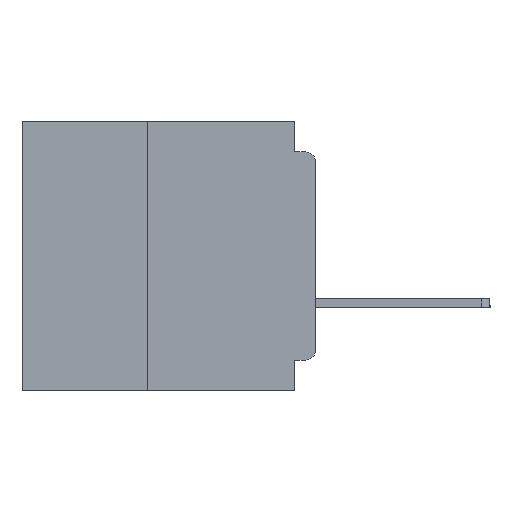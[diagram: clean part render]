
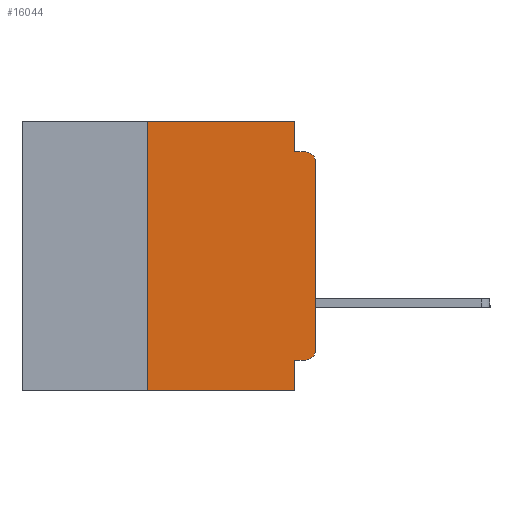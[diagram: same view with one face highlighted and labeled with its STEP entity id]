
A CAD part, left-side view. The second image highlights one B-rep face of the part: STEP entity #16044.
In plain terms, the highlighted planar face has unit normal (-1, 0, 0).
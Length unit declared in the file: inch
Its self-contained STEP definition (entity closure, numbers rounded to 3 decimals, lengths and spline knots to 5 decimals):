
#1748 = VECTOR ( 'NONE', #27761, 39.37008 ) ;
#2003 = CARTESIAN_POINT ( 'NONE',  ( 0., 0., -0.06 ) ) ;
#2313 = CARTESIAN_POINT ( 'NONE',  ( 0., 0.031, -0.4 ) ) ;
#3567 = VERTEX_POINT ( 'NONE', #19985 ) ;
#4343 = VECTOR ( 'NONE', #8860, 39.37008 ) ;
#4599 = VECTOR ( 'NONE', #20821, 39.37008 ) ;
#5480 = VERTEX_POINT ( 'NONE', #22633 ) ;
#5683 = LINE ( 'NONE', #7481, #4599 ) ;
#5689 = VERTEX_POINT ( 'NONE', #27144 ) ;
#6743 = DIRECTION ( 'NONE',  ( -1., 0., 0. ) ) ;
#7481 = CARTESIAN_POINT ( 'NONE',  ( 0., 0.25, -0.4 ) ) ;
#8166 = DIRECTION ( 'NONE',  ( 0., 1., 0. ) ) ;
#8509 = LINE ( 'NONE', #14944, #24227 ) ;
#8702 = EDGE_CURVE ( 'NONE', #5480, #36226, #37314, .T. ) ;
#8704 = VECTOR ( 'NONE', #33813, 39.37008 ) ;
#8860 = DIRECTION ( 'NONE',  ( 0., 0., -1. ) ) ;
#9264 = VECTOR ( 'NONE', #25425, 39.37008 ) ;
#10028 = CARTESIAN_POINT ( 'NONE',  ( 0., 0.031, -0.4 ) ) ;
#10109 = FACE_OUTER_BOUND ( 'NONE', #31327, .T. ) ;
#10285 = ORIENTED_EDGE ( 'NONE', *, *, #20589, .F. ) ;
#10366 = VERTEX_POINT ( 'NONE', #10028 ) ;
#10843 = AXIS2_PLACEMENT_3D ( 'NONE', #24779, #18190, #41308 ) ;
#11854 = CARTESIAN_POINT ( 'NONE',  ( 0., 0.031, -0.045 ) ) ;
#12310 = LINE ( 'NONE', #15456, #20171 ) ;
#12756 = EDGE_CURVE ( 'NONE', #31778, #36043, #36912, .T. ) ;
#12951 = ORIENTED_EDGE ( 'NONE', *, *, #12756, .T. ) ;
#13362 = LINE ( 'NONE', #2313, #4343 ) ;
#13823 = VERTEX_POINT ( 'NONE', #2003 ) ;
#14396 = ORIENTED_EDGE ( 'NONE', *, *, #25073, .T. ) ;
#14837 = PLANE ( 'NONE',  #10843 ) ;
#14944 = CARTESIAN_POINT ( 'NONE',  ( 0., 0., -0.355 ) ) ;
#15456 = CARTESIAN_POINT ( 'NONE',  ( 0., 0.437, -0.4 ) ) ;
#15842 = ORIENTED_EDGE ( 'NONE', *, *, #31777, .F. ) ;
#16030 = ORIENTED_EDGE ( 'NONE', *, *, #23142, .T. ) ;
#16044 = ADVANCED_FACE ( 'NONE', ( #10109 ), #14837, .F. ) ;
#18181 = LINE ( 'NONE', #41803, #9264 ) ;
#18190 = DIRECTION ( 'NONE',  ( 1., 0., 0. ) ) ;
#18360 = LINE ( 'NONE', #32692, #35008 ) ;
#19486 = EDGE_CURVE ( 'NONE', #13823, #29362, #39393, .T. ) ;
#19985 = CARTESIAN_POINT ( 'NONE',  ( 0., 0.031, -0.355 ) ) ;
#20169 = DIRECTION ( 'NONE',  ( -1., 0., 0. ) ) ;
#20171 = VECTOR ( 'NONE', #28774, 39.37008 ) ;
#20567 = CARTESIAN_POINT ( 'NONE',  ( 0., 0.031, 0. ) ) ;
#20589 = EDGE_CURVE ( 'NONE', #3567, #10366, #13362, .T. ) ;
#20821 = DIRECTION ( 'NONE',  ( 0., 0., 1. ) ) ;
#22382 = ORIENTED_EDGE ( 'NONE', *, *, #26221, .F. ) ;
#22633 = CARTESIAN_POINT ( 'NONE',  ( 0., 0.25, 0. ) ) ;
#23142 = EDGE_CURVE ( 'NONE', #36043, #13823, #18181, .T. ) ;
#23201 = ORIENTED_EDGE ( 'NONE', *, *, #8702, .F. ) ;
#23250 = CARTESIAN_POINT ( 'NONE',  ( 0., 0.031, 0. ) ) ;
#24227 = VECTOR ( 'NONE', #8166, 39.37008 ) ;
#24679 = ORIENTED_EDGE ( 'NONE', *, *, #19486, .T. ) ;
#24779 = CARTESIAN_POINT ( 'NONE',  ( 0., 0.437, 0. ) ) ;
#25073 = EDGE_CURVE ( 'NONE', #5689, #10366, #12310, .T. ) ;
#25425 = DIRECTION ( 'NONE',  ( 0., 0., 1. ) ) ;
#25524 = AXIS2_PLACEMENT_3D ( 'NONE', #26820, #6743, #30164 ) ;
#26221 = EDGE_CURVE ( 'NONE', #31778, #3567, #8509, .T. ) ;
#26269 = VERTEX_POINT ( 'NONE', #11854 ) ;
#26820 = CARTESIAN_POINT ( 'NONE',  ( 0., 0.015, -0.06 ) ) ;
#26828 = CARTESIAN_POINT ( 'NONE',  ( 0., 0.015, -0.045 ) ) ;
#27144 = CARTESIAN_POINT ( 'NONE',  ( 0., 0.25, -0.4 ) ) ;
#27761 = DIRECTION ( 'NONE',  ( 0., -1., 0. ) ) ;
#28774 = DIRECTION ( 'NONE',  ( 0., -1., 0. ) ) ;
#29362 = VERTEX_POINT ( 'NONE', #26828 ) ;
#29398 = ORIENTED_EDGE ( 'NONE', *, *, #41631, .F. ) ;
#29531 = EDGE_CURVE ( 'NONE', #5689, #5480, #5683, .T. ) ;
#29640 = AXIS2_PLACEMENT_3D ( 'NONE', #39954, #20169, #43210 ) ;
#30164 = DIRECTION ( 'NONE',  ( 0., 0., -1. ) ) ;
#31099 = CARTESIAN_POINT ( 'NONE',  ( 0., 0.437, 0. ) ) ;
#31327 = EDGE_LOOP ( 'NONE', ( #16030, #24679, #29398, #15842, #23201, #38214, #14396, #10285, #22382, #12951 ) ) ;
#31777 = EDGE_CURVE ( 'NONE', #36226, #26269, #42933, .T. ) ;
#31778 = VERTEX_POINT ( 'NONE', #40350 ) ;
#32692 = CARTESIAN_POINT ( 'NONE',  ( 0., 0., -0.045 ) ) ;
#33813 = DIRECTION ( 'NONE',  ( 0., 0., -1. ) ) ;
#35008 = VECTOR ( 'NONE', #35976, 39.37008 ) ;
#35976 = DIRECTION ( 'NONE',  ( 0., -1., 0. ) ) ;
#36043 = VERTEX_POINT ( 'NONE', #38853 ) ;
#36226 = VERTEX_POINT ( 'NONE', #23250 ) ;
#36912 = CIRCLE ( 'NONE', #29640, 0.015 ) ;
#37314 = LINE ( 'NONE', #31099, #1748 ) ;
#38214 = ORIENTED_EDGE ( 'NONE', *, *, #29531, .F. ) ;
#38853 = CARTESIAN_POINT ( 'NONE',  ( 0., 0., -0.34 ) ) ;
#39393 = CIRCLE ( 'NONE', #25524, 0.015 ) ;
#39954 = CARTESIAN_POINT ( 'NONE',  ( 0., 0.015, -0.34 ) ) ;
#40350 = CARTESIAN_POINT ( 'NONE',  ( 0., 0.015, -0.355 ) ) ;
#41308 = DIRECTION ( 'NONE',  ( 0., 0., -1. ) ) ;
#41631 = EDGE_CURVE ( 'NONE', #26269, #29362, #18360, .T. ) ;
#41803 = CARTESIAN_POINT ( 'NONE',  ( 0., 0., 0. ) ) ;
#42933 = LINE ( 'NONE', #20567, #8704 ) ;
#43210 = DIRECTION ( 'NONE',  ( 0., 0., -1. ) ) ;
